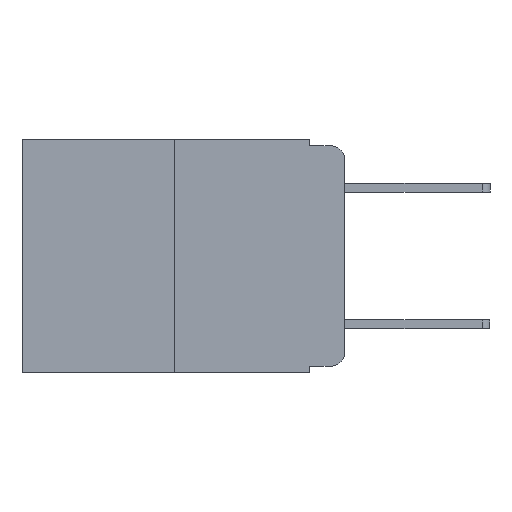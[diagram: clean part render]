
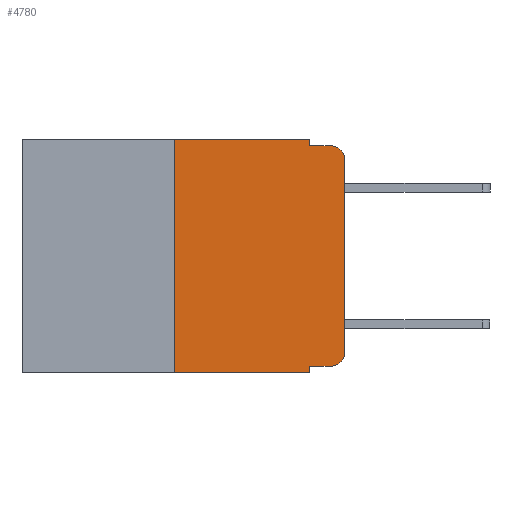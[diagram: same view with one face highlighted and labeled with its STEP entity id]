
A CAD part, left-side view. The second image highlights one B-rep face of the part: STEP entity #4780.
In plain terms, the highlighted planar face has unit normal (-1, 0, 0).
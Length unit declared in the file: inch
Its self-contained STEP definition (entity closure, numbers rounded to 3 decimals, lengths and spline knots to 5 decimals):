
#318 = LINE ( 'NONE', #16319, #9138 ) ;
#596 = AXIS2_PLACEMENT_3D ( 'NONE', #10922, #1125, #12482 ) ;
#610 = CIRCLE ( 'NONE', #6007, 0.02 ) ;
#861 = CARTESIAN_POINT ( 'NONE',  ( 0., 0.051, 0. ) ) ;
#892 = LINE ( 'NONE', #15526, #17330 ) ;
#948 = VECTOR ( 'NONE', #17338, 39.37008 ) ;
#1125 = DIRECTION ( 'NONE',  ( -1., 0., 0. ) ) ;
#1148 = CARTESIAN_POINT ( 'NONE',  ( 0., 0.051, 0. ) ) ;
#1241 = VERTEX_POINT ( 'NONE', #5638 ) ;
#1434 = LINE ( 'NONE', #15222, #5279 ) ;
#1488 = DIRECTION ( 'NONE',  ( 0., 0., -1. ) ) ;
#1952 = VECTOR ( 'NONE', #18500, 39.37008 ) ;
#1972 = EDGE_CURVE ( 'NONE', #13364, #6523, #20462, .T. ) ;
#2211 = ORIENTED_EDGE ( 'NONE', *, *, #19821, .T. ) ;
#2455 = LINE ( 'NONE', #1148, #1952 ) ;
#2799 = DIRECTION ( 'NONE',  ( 1., 0., 0. ) ) ;
#2946 = DIRECTION ( 'NONE',  ( 0., -1., 0. ) ) ;
#3322 = EDGE_LOOP ( 'NONE', ( #8058, #17265, #12049, #7694, #14430, #13248, #6827, #7840, #5526, #2211 ) ) ;
#3397 = EDGE_CURVE ( 'NONE', #1241, #15566, #14543, .T. ) ;
#3434 = CARTESIAN_POINT ( 'NONE',  ( 0., 0.051, -0.01 ) ) ;
#4217 = DIRECTION ( 'NONE',  ( 0., 0., -1. ) ) ;
#4582 = VECTOR ( 'NONE', #4217, 39.37008 ) ;
#4601 = VERTEX_POINT ( 'NONE', #14988 ) ;
#4780 = ADVANCED_FACE ( 'NONE', ( #11151 ), #18472, .F. ) ;
#4840 = EDGE_CURVE ( 'NONE', #4601, #18817, #892, .T. ) ;
#5074 = DIRECTION ( 'NONE',  ( 0., -1., 0. ) ) ;
#5218 = CARTESIAN_POINT ( 'NONE',  ( 0., 0.473, -0.343 ) ) ;
#5223 = CARTESIAN_POINT ( 'NONE',  ( 0., 0.02, -0.01 ) ) ;
#5245 = EDGE_CURVE ( 'NONE', #6463, #13364, #1434, .T. ) ;
#5256 = CARTESIAN_POINT ( 'NONE',  ( 0., 0.051, -0.01 ) ) ;
#5279 = VECTOR ( 'NONE', #9089, 39.37008 ) ;
#5526 = ORIENTED_EDGE ( 'NONE', *, *, #4840, .T. ) ;
#5638 = CARTESIAN_POINT ( 'NONE',  ( 0., 0.25, -0.343 ) ) ;
#6007 = AXIS2_PLACEMENT_3D ( 'NONE', #20274, #11257, #1488 ) ;
#6039 = CARTESIAN_POINT ( 'NONE',  ( 0., 0.473, 0. ) ) ;
#6463 = VERTEX_POINT ( 'NONE', #18987 ) ;
#6523 = VERTEX_POINT ( 'NONE', #5223 ) ;
#6696 = VECTOR ( 'NONE', #16260, 39.37008 ) ;
#6827 = ORIENTED_EDGE ( 'NONE', *, *, #3397, .T. ) ;
#7467 = EDGE_CURVE ( 'NONE', #12931, #15997, #2455, .T. ) ;
#7694 = ORIENTED_EDGE ( 'NONE', *, *, #7467, .F. ) ;
#7840 = ORIENTED_EDGE ( 'NONE', *, *, #11756, .F. ) ;
#8058 = ORIENTED_EDGE ( 'NONE', *, *, #5245, .T. ) ;
#8255 = AXIS2_PLACEMENT_3D ( 'NONE', #6039, #2799, #13986 ) ;
#9089 = DIRECTION ( 'NONE',  ( 0., 0., 1. ) ) ;
#9138 = VECTOR ( 'NONE', #19291, 39.37008 ) ;
#9634 = EDGE_CURVE ( 'NONE', #15997, #6523, #16766, .T. ) ;
#9701 = CARTESIAN_POINT ( 'NONE',  ( 0., 0.25, 0. ) ) ;
#9707 = LINE ( 'NONE', #9701, #948 ) ;
#10622 = CARTESIAN_POINT ( 'NONE',  ( 0., 0.051, -0.343 ) ) ;
#10682 = VERTEX_POINT ( 'NONE', #20175 ) ;
#10922 = CARTESIAN_POINT ( 'NONE',  ( 0., 0.02, -0.03 ) ) ;
#11151 = FACE_OUTER_BOUND ( 'NONE', #3322, .T. ) ;
#11257 = DIRECTION ( 'NONE',  ( -1., 0., 0. ) ) ;
#11756 = EDGE_CURVE ( 'NONE', #4601, #15566, #17129, .T. ) ;
#11900 = CARTESIAN_POINT ( 'NONE',  ( 0., 0.02, -0.333 ) ) ;
#12049 = ORIENTED_EDGE ( 'NONE', *, *, #9634, .F. ) ;
#12482 = DIRECTION ( 'NONE',  ( 0., 0., -1. ) ) ;
#12931 = VERTEX_POINT ( 'NONE', #13476 ) ;
#13248 = ORIENTED_EDGE ( 'NONE', *, *, #15834, .F. ) ;
#13364 = VERTEX_POINT ( 'NONE', #17492 ) ;
#13476 = CARTESIAN_POINT ( 'NONE',  ( 0., 0.051, 0. ) ) ;
#13986 = DIRECTION ( 'NONE',  ( 0., 0., -1. ) ) ;
#14430 = ORIENTED_EDGE ( 'NONE', *, *, #20049, .F. ) ;
#14543 = LINE ( 'NONE', #5218, #6696 ) ;
#14988 = CARTESIAN_POINT ( 'NONE',  ( 0., 0.051, -0.333 ) ) ;
#15222 = CARTESIAN_POINT ( 'NONE',  ( 0., 0., 0. ) ) ;
#15526 = CARTESIAN_POINT ( 'NONE',  ( 0., 0.051, -0.333 ) ) ;
#15566 = VERTEX_POINT ( 'NONE', #10622 ) ;
#15834 = EDGE_CURVE ( 'NONE', #1241, #10682, #9707, .T. ) ;
#15997 = VERTEX_POINT ( 'NONE', #5256 ) ;
#16260 = DIRECTION ( 'NONE',  ( 0., -1., 0. ) ) ;
#16319 = CARTESIAN_POINT ( 'NONE',  ( 0., 0.473, 0. ) ) ;
#16766 = LINE ( 'NONE', #3434, #18841 ) ;
#17129 = LINE ( 'NONE', #861, #4582 ) ;
#17265 = ORIENTED_EDGE ( 'NONE', *, *, #1972, .T. ) ;
#17330 = VECTOR ( 'NONE', #2946, 39.37008 ) ;
#17338 = DIRECTION ( 'NONE',  ( 0., 0., 1. ) ) ;
#17492 = CARTESIAN_POINT ( 'NONE',  ( 0., 0., -0.03 ) ) ;
#18472 = PLANE ( 'NONE',  #8255 ) ;
#18500 = DIRECTION ( 'NONE',  ( 0., 0., -1. ) ) ;
#18817 = VERTEX_POINT ( 'NONE', #11900 ) ;
#18841 = VECTOR ( 'NONE', #5074, 39.37008 ) ;
#18987 = CARTESIAN_POINT ( 'NONE',  ( 0., 0., -0.313 ) ) ;
#19291 = DIRECTION ( 'NONE',  ( 0., -1., 0. ) ) ;
#19821 = EDGE_CURVE ( 'NONE', #18817, #6463, #610, .T. ) ;
#20049 = EDGE_CURVE ( 'NONE', #10682, #12931, #318, .T. ) ;
#20175 = CARTESIAN_POINT ( 'NONE',  ( 0., 0.25, 0. ) ) ;
#20274 = CARTESIAN_POINT ( 'NONE',  ( 0., 0.02, -0.313 ) ) ;
#20462 = CIRCLE ( 'NONE', #596, 0.02 ) ;
